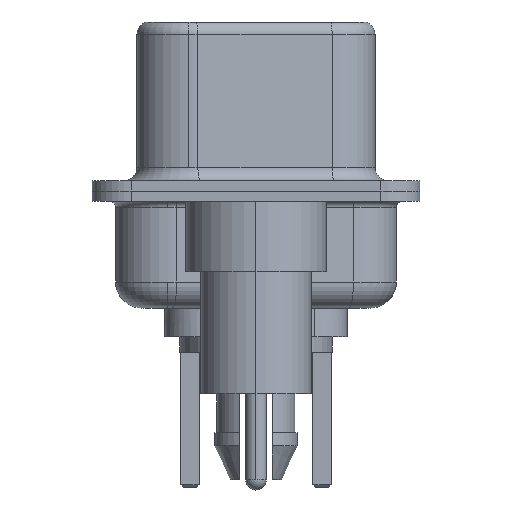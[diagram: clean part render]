
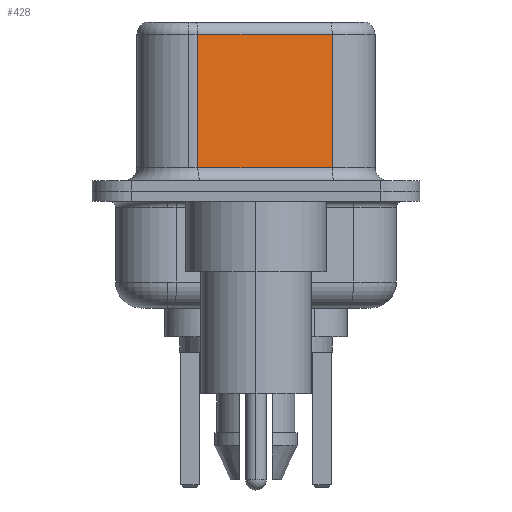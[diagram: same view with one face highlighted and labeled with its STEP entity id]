
A CAD part, left-side view. The second image highlights one B-rep face of the part: STEP entity #428.
In plain terms, the highlighted planar face has unit normal (-0.985, -0.174, 0).
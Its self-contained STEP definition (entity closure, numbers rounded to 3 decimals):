
#428 = ADVANCED_FACE ( 'NONE', ( #10944 ), #13478, .F. ) ;
#1987 = VECTOR ( 'NONE', #15738, 1000. ) ;
#2743 = CARTESIAN_POINT ( 'NONE',  ( 4.58, -2.927, 6.52 ) ) ;
#3418 = ORIENTED_EDGE ( 'NONE', *, *, #16404, .T. ) ;
#4548 = EDGE_CURVE ( 'NONE', #6217, #14363, #12972, .T. ) ;
#4972 = CARTESIAN_POINT ( 'NONE',  ( 4.58, -2.927, 6.52 ) ) ;
#4978 = VERTEX_POINT ( 'NONE', #6727 ) ;
#5229 = DIRECTION ( 'NONE',  ( 0.174, -0.985, 0. ) ) ;
#5454 = ORIENTED_EDGE ( 'NONE', *, *, #16102, .T. ) ;
#6060 = DIRECTION ( 'NONE',  ( -0.174, 0.985, 0. ) ) ;
#6217 = VERTEX_POINT ( 'NONE', #11778 ) ;
#6727 = CARTESIAN_POINT ( 'NONE',  ( 3.67, 2.233, 6.02 ) ) ;
#6898 = LINE ( 'NONE', #16334, #7367 ) ;
#7345 = CARTESIAN_POINT ( 'NONE',  ( 4.58, -2.927, 0.9 ) ) ;
#7367 = VECTOR ( 'NONE', #6060, 1000. ) ;
#9422 = DIRECTION ( 'NONE',  ( 0., 0., -1. ) ) ;
#9522 = VECTOR ( 'NONE', #9422, 1000. ) ;
#10582 = LINE ( 'NONE', #12422, #17926 ) ;
#10944 = FACE_OUTER_BOUND ( 'NONE', #11529, .T. ) ;
#11376 = CARTESIAN_POINT ( 'NONE',  ( 3.67, 2.233, 6.52 ) ) ;
#11529 = EDGE_LOOP ( 'NONE', ( #13084, #5454, #16245, #3418 ) ) ;
#11778 = CARTESIAN_POINT ( 'NONE',  ( 4.58, -2.927, 6.02 ) ) ;
#12422 = CARTESIAN_POINT ( 'NONE',  ( 4.58, -2.927, 0.9 ) ) ;
#12972 = LINE ( 'NONE', #2743, #9522 ) ;
#13084 = ORIENTED_EDGE ( 'NONE', *, *, #4548, .F. ) ;
#13478 = PLANE ( 'NONE',  #15053 ) ;
#14363 = VERTEX_POINT ( 'NONE', #7345 ) ;
#15053 = AXIS2_PLACEMENT_3D ( 'NONE', #4972, #17020, #17039 ) ;
#15616 = CARTESIAN_POINT ( 'NONE',  ( 3.67, 2.233, 0.9 ) ) ;
#15738 = DIRECTION ( 'NONE',  ( 0., 0., -1. ) ) ;
#16102 = EDGE_CURVE ( 'NONE', #6217, #4978, #6898, .T. ) ;
#16245 = ORIENTED_EDGE ( 'NONE', *, *, #17587, .T. ) ;
#16334 = CARTESIAN_POINT ( 'NONE',  ( 4.58, -2.927, 6.02 ) ) ;
#16404 = EDGE_CURVE ( 'NONE', #17512, #14363, #10582, .T. ) ;
#17020 = DIRECTION ( 'NONE',  ( 0.985, 0.174, 0. ) ) ;
#17039 = DIRECTION ( 'NONE',  ( -0.174, 0.985, 0. ) ) ;
#17512 = VERTEX_POINT ( 'NONE', #15616 ) ;
#17587 = EDGE_CURVE ( 'NONE', #4978, #17512, #17693, .T. ) ;
#17693 = LINE ( 'NONE', #11376, #1987 ) ;
#17926 = VECTOR ( 'NONE', #5229, 1000. ) ;
